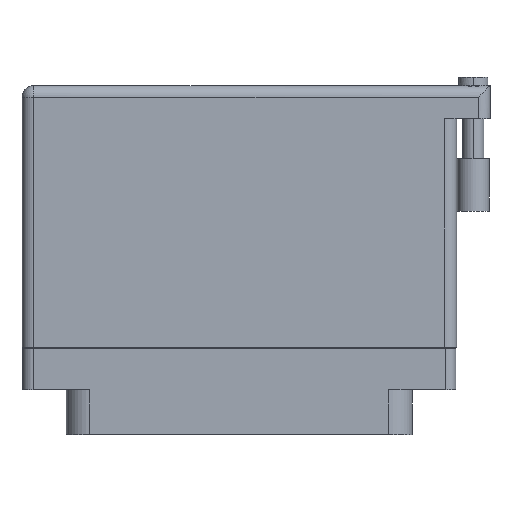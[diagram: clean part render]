
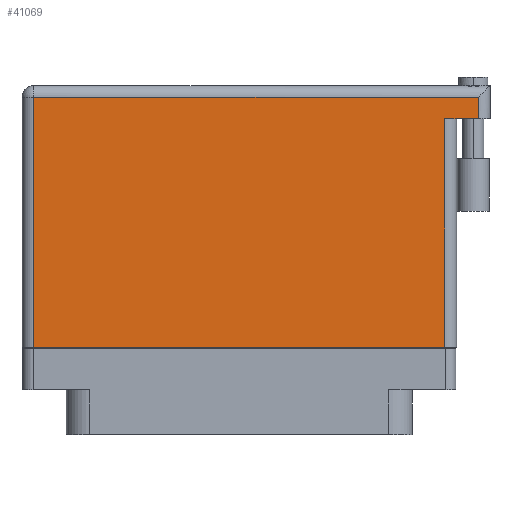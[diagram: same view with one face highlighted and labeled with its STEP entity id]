
A CAD part, front view. The second image highlights one B-rep face of the part: STEP entity #41069.
In plain terms, the highlighted face is planar.
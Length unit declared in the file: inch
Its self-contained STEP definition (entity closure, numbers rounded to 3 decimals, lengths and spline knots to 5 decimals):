
#509 = CARTESIAN_POINT ( 'NONE',  ( 1.43, 1.466, 0.4495 ) ) ;
#1402 = EDGE_LOOP ( 'NONE', ( #26940, #31020, #7487, #35654, #28865, #14224 ) ) ;
#1922 = DIRECTION ( 'NONE',  ( 0., -1., 0. ) ) ;
#2129 = EDGE_CURVE ( 'NONE', #37671, #14533, #24763, .T. ) ;
#3680 = CARTESIAN_POINT ( 'NONE',  ( 1.23, -0.1, 0.4495 ) ) ;
#4619 = LINE ( 'NONE', #509, #38421 ) ;
#5071 = CARTESIAN_POINT ( 'NONE',  ( -1.3, 1.396, 0.4495 ) ) ;
#6311 = EDGE_CURVE ( 'NONE', #20197, #40936, #10416, .T. ) ;
#6887 = LINE ( 'NONE', #34333, #12058 ) ;
#7487 = ORIENTED_EDGE ( 'NONE', *, *, #6311, .F. ) ;
#8684 = LINE ( 'NONE', #21821, #34139 ) ;
#9335 = CARTESIAN_POINT ( 'NONE',  ( 1.23, 1.269, 0.4495 ) ) ;
#9494 = DIRECTION ( 'NONE',  ( -1., 0., 0. ) ) ;
#10416 = LINE ( 'NONE', #29231, #37929 ) ;
#10486 = CARTESIAN_POINT ( 'NONE',  ( -1.3, 1.466, 0.4495 ) ) ;
#11055 = VERTEX_POINT ( 'NONE', #34733 ) ;
#12058 = VECTOR ( 'NONE', #20867, 39.37008 ) ;
#13372 = EDGE_CURVE ( 'NONE', #20197, #37671, #4619, .T. ) ;
#13937 = DIRECTION ( 'NONE',  ( -1., 0., 0. ) ) ;
#14224 = ORIENTED_EDGE ( 'NONE', *, *, #34045, .T. ) ;
#14533 = VERTEX_POINT ( 'NONE', #24634 ) ;
#18422 = DIRECTION ( 'NONE',  ( -1., 0., 0. ) ) ;
#19762 = EDGE_CURVE ( 'NONE', #11055, #40194, #25249, .T. ) ;
#20197 = VERTEX_POINT ( 'NONE', #39071 ) ;
#20569 = DIRECTION ( 'NONE',  ( 0., 1., 0. ) ) ;
#20652 = DIRECTION ( 'NONE',  ( 0., 0., -1. ) ) ;
#20867 = DIRECTION ( 'NONE',  ( 0., 1., 0. ) ) ;
#21821 = CARTESIAN_POINT ( 'NONE',  ( -1.23, -0.1, 0.4495 ) ) ;
#23724 = EDGE_CURVE ( 'NONE', #40194, #40936, #6887, .T. ) ;
#23768 = VECTOR ( 'NONE', #18422, 39.37008 ) ;
#24634 = CARTESIAN_POINT ( 'NONE',  ( -1.23, 1.396, 0.4495 ) ) ;
#24763 = LINE ( 'NONE', #5071, #23768 ) ;
#25249 = LINE ( 'NONE', #38406, #37680 ) ;
#26940 = ORIENTED_EDGE ( 'NONE', *, *, #19762, .T. ) ;
#28865 = ORIENTED_EDGE ( 'NONE', *, *, #2129, .T. ) ;
#29231 = CARTESIAN_POINT ( 'NONE',  ( 1.5, 1.269, 0.4495 ) ) ;
#29470 = CARTESIAN_POINT ( 'NONE',  ( 1.43, 1.396, 0.4495 ) ) ;
#31020 = ORIENTED_EDGE ( 'NONE', *, *, #23724, .T. ) ;
#33522 = FACE_OUTER_BOUND ( 'NONE', #1402, .T. ) ;
#34045 = EDGE_CURVE ( 'NONE', #14533, #11055, #8684, .T. ) ;
#34139 = VECTOR ( 'NONE', #1922, 39.37008 ) ;
#34333 = CARTESIAN_POINT ( 'NONE',  ( 1.23, 1.269, 0.4495 ) ) ;
#34733 = CARTESIAN_POINT ( 'NONE',  ( -1.23, -0.1, 0.4495 ) ) ;
#35654 = ORIENTED_EDGE ( 'NONE', *, *, #13372, .T. ) ;
#37671 = VERTEX_POINT ( 'NONE', #29470 ) ;
#37680 = VECTOR ( 'NONE', #38543, 39.37008 ) ;
#37929 = VECTOR ( 'NONE', #9494, 39.37008 ) ;
#38406 = CARTESIAN_POINT ( 'NONE',  ( -1.3, -0.1, 0.4495 ) ) ;
#38421 = VECTOR ( 'NONE', #20569, 39.37008 ) ;
#38543 = DIRECTION ( 'NONE',  ( 1., 0., 0. ) ) ;
#39071 = CARTESIAN_POINT ( 'NONE',  ( 1.43, 1.269, 0.4495 ) ) ;
#39371 = AXIS2_PLACEMENT_3D ( 'NONE', #10486, #20652, #13937 ) ;
#40194 = VERTEX_POINT ( 'NONE', #3680 ) ;
#40410 = PLANE ( 'NONE',  #39371 ) ;
#40936 = VERTEX_POINT ( 'NONE', #9335 ) ;
#41069 = ADVANCED_FACE ( 'NONE', ( #33522 ), #40410, .F. ) ;
